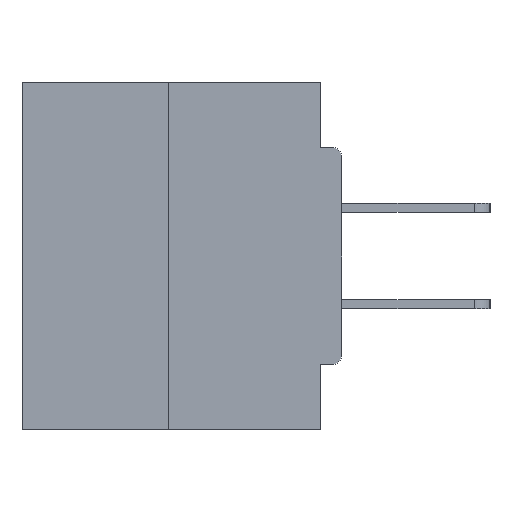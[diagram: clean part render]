
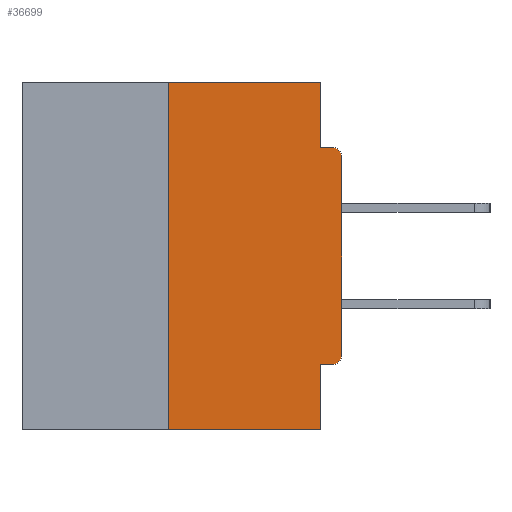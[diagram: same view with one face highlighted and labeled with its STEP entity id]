
A CAD part, left-side view. The second image highlights one B-rep face of the part: STEP entity #36699.
In plain terms, the highlighted planar face has unit normal (-1, 0, 0).
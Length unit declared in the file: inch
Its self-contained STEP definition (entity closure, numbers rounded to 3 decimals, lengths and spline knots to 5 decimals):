
#194 = ORIENTED_EDGE ( 'NONE', *, *, #13804, .T. ) ;
#578 = VERTEX_POINT ( 'NONE', #31167 ) ;
#718 = CARTESIAN_POINT ( 'NONE',  ( 0., 0., -0.0935 ) ) ;
#1397 = CARTESIAN_POINT ( 'NONE',  ( 0., 0., -0.1085 ) ) ;
#2165 = ORIENTED_EDGE ( 'NONE', *, *, #45806, .F. ) ;
#2578 = VERTEX_POINT ( 'NONE', #27797 ) ;
#3330 = CARTESIAN_POINT ( 'NONE',  ( 0., 0.46, -0.5 ) ) ;
#3383 = VERTEX_POINT ( 'NONE', #23890 ) ;
#4112 = DIRECTION ( 'NONE',  ( 0., 0., -1. ) ) ;
#4696 = CARTESIAN_POINT ( 'NONE',  ( 0., 0.46, 0. ) ) ;
#6241 = DIRECTION ( 'NONE',  ( 1., 0., 0. ) ) ;
#6669 = DIRECTION ( 'NONE',  ( 0., 1., 0. ) ) ;
#8298 = CIRCLE ( 'NONE', #27694, 0.015 ) ;
#9030 = EDGE_CURVE ( 'NONE', #15456, #2578, #42349, .T. ) ;
#9142 = VECTOR ( 'NONE', #37978, 39.37008 ) ;
#9754 = CARTESIAN_POINT ( 'NONE',  ( 0., 0.031, -0.5 ) ) ;
#11022 = DIRECTION ( 'NONE',  ( -1., 0., 0. ) ) ;
#11723 = VERTEX_POINT ( 'NONE', #19874 ) ;
#11796 = EDGE_CURVE ( 'NONE', #20593, #578, #30208, .T. ) ;
#12005 = VECTOR ( 'NONE', #39756, 39.37008 ) ;
#12399 = VECTOR ( 'NONE', #33113, 39.37008 ) ;
#13114 = ORIENTED_EDGE ( 'NONE', *, *, #44378, .T. ) ;
#13729 = CARTESIAN_POINT ( 'NONE',  ( 0., 0., -0.4065 ) ) ;
#13804 = EDGE_CURVE ( 'NONE', #22620, #15456, #18713, .T. ) ;
#14247 = ORIENTED_EDGE ( 'NONE', *, *, #21645, .T. ) ;
#14362 = DIRECTION ( 'NONE',  ( 0., 0., -1. ) ) ;
#15125 = ORIENTED_EDGE ( 'NONE', *, *, #9030, .T. ) ;
#15456 = VERTEX_POINT ( 'NONE', #1397 ) ;
#15533 = DIRECTION ( 'NONE',  ( -1., 0., 0. ) ) ;
#16016 = EDGE_CURVE ( 'NONE', #21598, #11723, #29325, .T. ) ;
#16484 = CARTESIAN_POINT ( 'NONE',  ( 0., 0., 0. ) ) ;
#17110 = CARTESIAN_POINT ( 'NONE',  ( 0., 0.031, -0.5 ) ) ;
#17153 = DIRECTION ( 'NONE',  ( 0., 0., -1. ) ) ;
#17679 = LINE ( 'NONE', #3330, #12005 ) ;
#17694 = CARTESIAN_POINT ( 'NONE',  ( 0., 0.031, 0. ) ) ;
#18713 = LINE ( 'NONE', #16484, #9142 ) ;
#18865 = DIRECTION ( 'NONE',  ( 0., 0., -1. ) ) ;
#19874 = CARTESIAN_POINT ( 'NONE',  ( 0., 0.031, -0.4065 ) ) ;
#19972 = CARTESIAN_POINT ( 'NONE',  ( 0., 0., -0.3915 ) ) ;
#20593 = VERTEX_POINT ( 'NONE', #28570 ) ;
#20600 = CARTESIAN_POINT ( 'NONE',  ( 0., 0.46, 0. ) ) ;
#21598 = VERTEX_POINT ( 'NONE', #22792 ) ;
#21645 = EDGE_CURVE ( 'NONE', #21598, #22620, #8298, .T. ) ;
#22620 = VERTEX_POINT ( 'NONE', #19972 ) ;
#22792 = CARTESIAN_POINT ( 'NONE',  ( 0., 0.015, -0.4065 ) ) ;
#23890 = CARTESIAN_POINT ( 'NONE',  ( 0., 0.25, -0.5 ) ) ;
#24206 = VECTOR ( 'NONE', #17153, 39.37008 ) ;
#24300 = ORIENTED_EDGE ( 'NONE', *, *, #16016, .F. ) ;
#24547 = ORIENTED_EDGE ( 'NONE', *, *, #11796, .F. ) ;
#24805 = ORIENTED_EDGE ( 'NONE', *, *, #33804, .F. ) ;
#25920 = VECTOR ( 'NONE', #6669, 39.37008 ) ;
#26858 = ORIENTED_EDGE ( 'NONE', *, *, #43168, .F. ) ;
#26932 = VECTOR ( 'NONE', #37618, 39.37008 ) ;
#27155 = EDGE_LOOP ( 'NONE', ( #26858, #24805, #13114, #33618, #24300, #14247, #194, #15125, #2165, #24547 ) ) ;
#27694 = AXIS2_PLACEMENT_3D ( 'NONE', #29746, #15533, #18865 ) ;
#27797 = CARTESIAN_POINT ( 'NONE',  ( 0., 0.015, -0.0935 ) ) ;
#28388 = CARTESIAN_POINT ( 'NONE',  ( 0., 0.25, 0. ) ) ;
#28570 = CARTESIAN_POINT ( 'NONE',  ( 0., 0.031, 0. ) ) ;
#29325 = LINE ( 'NONE', #13729, #25920 ) ;
#29746 = CARTESIAN_POINT ( 'NONE',  ( 0., 0.015, -0.3915 ) ) ;
#30058 = DIRECTION ( 'NONE',  ( 0., -1., 0. ) ) ;
#30208 = LINE ( 'NONE', #17694, #42678 ) ;
#31167 = CARTESIAN_POINT ( 'NONE',  ( 0., 0.031, -0.0935 ) ) ;
#33113 = DIRECTION ( 'NONE',  ( 0., -1., 0. ) ) ;
#33435 = FACE_OUTER_BOUND ( 'NONE', #27155, .T. ) ;
#33618 = ORIENTED_EDGE ( 'NONE', *, *, #40262, .F. ) ;
#33804 = EDGE_CURVE ( 'NONE', #3383, #35923, #35396, .T. ) ;
#34144 = CARTESIAN_POINT ( 'NONE',  ( 0., 0.25, 0. ) ) ;
#34648 = VECTOR ( 'NONE', #30058, 39.37008 ) ;
#34933 = DIRECTION ( 'NONE',  ( 0., 0., -1. ) ) ;
#35009 = LINE ( 'NONE', #718, #12399 ) ;
#35396 = LINE ( 'NONE', #34144, #26932 ) ;
#35923 = VERTEX_POINT ( 'NONE', #28388 ) ;
#36699 = ADVANCED_FACE ( 'NONE', ( #33435 ), #38587, .F. ) ;
#37618 = DIRECTION ( 'NONE',  ( 0., 0., 1. ) ) ;
#37978 = DIRECTION ( 'NONE',  ( 0., 0., 1. ) ) ;
#38587 = PLANE ( 'NONE',  #41174 ) ;
#39756 = DIRECTION ( 'NONE',  ( 0., -1., 0. ) ) ;
#40262 = EDGE_CURVE ( 'NONE', #11723, #41832, #43458, .T. ) ;
#41174 = AXIS2_PLACEMENT_3D ( 'NONE', #20600, #6241, #34933 ) ;
#41832 = VERTEX_POINT ( 'NONE', #17110 ) ;
#42349 = CIRCLE ( 'NONE', #43824, 0.015 ) ;
#42678 = VECTOR ( 'NONE', #14362, 39.37008 ) ;
#43168 = EDGE_CURVE ( 'NONE', #35923, #20593, #44309, .T. ) ;
#43458 = LINE ( 'NONE', #9754, #24206 ) ;
#43550 = CARTESIAN_POINT ( 'NONE',  ( 0., 0.015, -0.1085 ) ) ;
#43824 = AXIS2_PLACEMENT_3D ( 'NONE', #43550, #11022, #4112 ) ;
#44309 = LINE ( 'NONE', #4696, #34648 ) ;
#44378 = EDGE_CURVE ( 'NONE', #3383, #41832, #17679, .T. ) ;
#45806 = EDGE_CURVE ( 'NONE', #578, #2578, #35009, .T. ) ;
